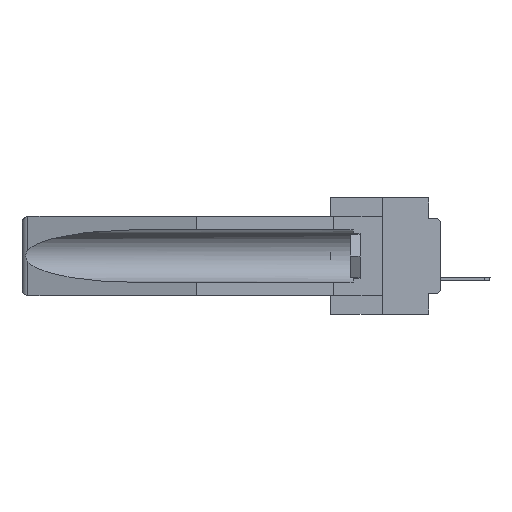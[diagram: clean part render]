
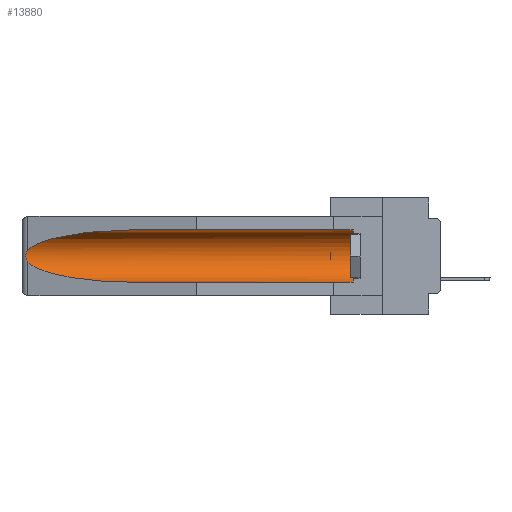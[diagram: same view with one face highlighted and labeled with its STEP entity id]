
A CAD part, left-side view. The second image highlights one B-rep face of the part: STEP entity #13880.
In plain terms, the highlighted cylindrical face has radius 2.857 mm (diameter 5.715 mm), a partial arc.
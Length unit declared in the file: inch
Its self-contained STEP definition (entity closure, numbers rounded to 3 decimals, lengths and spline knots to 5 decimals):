
#2899 = CARTESIAN_POINT ( 'NONE',  ( 0.26654, 1.53092, -0.15636 ) ) ;
#3730 = ORIENTED_EDGE ( 'NONE', *, *, #39658, .T. ) ;
#3812 = CARTESIAN_POINT ( 'NONE',  ( 0.155, -0.30754, -0.284 ) ) ;
#4003 = CARTESIAN_POINT ( 'NONE',  ( 0.155, 0.126, -0.1715 ) ) ;
#5681 = ORIENTED_EDGE ( 'NONE', *, *, #24620, .T. ) ;
#5721 = CARTESIAN_POINT ( 'NONE',  ( 0.2673, 1.53269, -0.17917 ) ) ;
#6647 = VERTEX_POINT ( 'NONE', #15003 ) ;
#6692 = FACE_OUTER_BOUND ( 'NONE', #24345, .T. ) ;
#7071 = VERTEX_POINT ( 'NONE', #22682 ) ;
#7233 = DIRECTION ( 'NONE',  ( 0., 0., 1. ) ) ;
#7911 = VECTOR ( 'NONE', #9457, 39.37008 ) ;
#8857 = VERTEX_POINT ( 'NONE', #20600 ) ;
#9457 = DIRECTION ( 'NONE',  ( 0., 1., 0. ) ) ;
#9599 =( BOUNDED_CURVE ( )  B_SPLINE_CURVE ( 3, ( #34732, #25431, #34131, #37180 ),
 .UNSPECIFIED., .F., .T. ) 
 B_SPLINE_CURVE_WITH_KNOTS ( ( 4, 4 ),
 ( 4.71239, 6.08839 ),
 .UNSPECIFIED. ) 
 CURVE ( )  GEOMETRIC_REPRESENTATION_ITEM ( )  RATIONAL_B_SPLINE_CURVE ( ( 1., 0.848, 0.848, 1. ) ) 
 REPRESENTATION_ITEM ( '' )  );
#9711 = EDGE_CURVE ( 'NONE', #28031, #6647, #16634, .T. ) ;
#10058 = DIRECTION ( 'NONE',  ( 0., -1., 0. ) ) ;
#12958 = VERTEX_POINT ( 'NONE', #27577 ) ;
#13326 = DIRECTION ( 'NONE',  ( 0., 1., 0. ) ) ;
#13880 = ADVANCED_FACE ( 'NONE', ( #6692 ), #16547, .F. ) ;
#14579 = CARTESIAN_POINT ( 'NONE',  ( 0.26597, 1.5296, -0.19026 ) ) ;
#14958 = VERTEX_POINT ( 'NONE', #20837 ) ;
#14965 = CARTESIAN_POINT ( 'NONE',  ( 0.26537, 1.52718, -0.14972 ) ) ;
#15003 = CARTESIAN_POINT ( 'NONE',  ( 0.26537, 1.52718, -0.19328 ) ) ;
#16547 = CYLINDRICAL_SURFACE ( 'NONE', #31322, 0.1125 ) ;
#16634 = B_SPLINE_CURVE_WITH_KNOTS ( 'NONE', 3,
 ( #14965, #39653, #2899, #27715, #36206, #24475, #5721, #18210, #14579, #30339 ),
 .UNSPECIFIED., .F., .F.,
 ( 4, 2, 2, 2, 4 ),
 ( 0., 0.00029, 0.00058, 0.00087, 0.00117 ),
 .UNSPECIFIED. ) ;
#16769 = CARTESIAN_POINT ( 'NONE',  ( 0.25451, 1.48313, -0.24835 ) ) ;
#17550 = CARTESIAN_POINT ( 'NONE',  ( 0.155, 1.07973, -0.284 ) ) ;
#18210 = CARTESIAN_POINT ( 'NONE',  ( 0.26655, 1.53094, -0.18657 ) ) ;
#19014 = AXIS2_PLACEMENT_3D ( 'NONE', #4003, #10058, #7233 ) ;
#19797 = DIRECTION ( 'NONE',  ( 0., 0., 1. ) ) ;
#19819 = EDGE_CURVE ( 'NONE', #6647, #12958, #28936, .T. ) ;
#20600 = CARTESIAN_POINT ( 'NONE',  ( 0.155, 0.126, -0.059 ) ) ;
#20837 = CARTESIAN_POINT ( 'NONE',  ( 0.155, 0.126, -0.284 ) ) ;
#21267 = ORIENTED_EDGE ( 'NONE', *, *, #19819, .T. ) ;
#21851 = ORIENTED_EDGE ( 'NONE', *, *, #25089, .F. ) ;
#22682 = CARTESIAN_POINT ( 'NONE',  ( 0.155, 1.07973, -0.059 ) ) ;
#24345 = EDGE_LOOP ( 'NONE', ( #29338, #39216, #21267, #21851, #3730, #5681 ) ) ;
#24475 = CARTESIAN_POINT ( 'NONE',  ( 0.2675, 1.53308, -0.17534 ) ) ;
#24620 = EDGE_CURVE ( 'NONE', #8857, #7071, #30903, .T. ) ;
#24633 = EDGE_CURVE ( 'NONE', #7071, #28031, #9599, .T. ) ;
#25089 = EDGE_CURVE ( 'NONE', #14958, #12958, #31462, .T. ) ;
#25431 = CARTESIAN_POINT ( 'NONE',  ( 0.21114, 1.30732, -0.059 ) ) ;
#27180 = CARTESIAN_POINT ( 'NONE',  ( 0.26537, 1.52718, -0.14972 ) ) ;
#27577 = CARTESIAN_POINT ( 'NONE',  ( 0.155, 1.07973, -0.284 ) ) ;
#27715 = CARTESIAN_POINT ( 'NONE',  ( 0.2673, 1.5327, -0.16383 ) ) ;
#28031 = VERTEX_POINT ( 'NONE', #27180 ) ;
#28936 =( BOUNDED_CURVE ( )  B_SPLINE_CURVE ( 3, ( #35358, #16769, #35759, #17550 ),
 .UNSPECIFIED., .F., .T. ) 
 B_SPLINE_CURVE_WITH_KNOTS ( ( 4, 4 ),
 ( 0.1948, 1.5708 ),
 .UNSPECIFIED. ) 
 CURVE ( )  GEOMETRIC_REPRESENTATION_ITEM ( )  RATIONAL_B_SPLINE_CURVE ( ( 1., 0.848, 0.848, 1. ) ) 
 REPRESENTATION_ITEM ( '' )  );
#29338 = ORIENTED_EDGE ( 'NONE', *, *, #24633, .T. ) ;
#30339 = CARTESIAN_POINT ( 'NONE',  ( 0.26537, 1.52718, -0.19328 ) ) ;
#30903 = LINE ( 'NONE', #31701, #36847 ) ;
#31322 = AXIS2_PLACEMENT_3D ( 'NONE', #38177, #34933, #19797 ) ;
#31462 = LINE ( 'NONE', #3812, #7911 ) ;
#31701 = CARTESIAN_POINT ( 'NONE',  ( 0.155, -0.30754, -0.059 ) ) ;
#34131 = CARTESIAN_POINT ( 'NONE',  ( 0.25451, 1.48313, -0.09465 ) ) ;
#34732 = CARTESIAN_POINT ( 'NONE',  ( 0.155, 1.07973, -0.059 ) ) ;
#34933 = DIRECTION ( 'NONE',  ( 0., 1., 0. ) ) ;
#35358 = CARTESIAN_POINT ( 'NONE',  ( 0.26537, 1.52718, -0.19328 ) ) ;
#35759 = CARTESIAN_POINT ( 'NONE',  ( 0.21114, 1.30732, -0.284 ) ) ;
#36206 = CARTESIAN_POINT ( 'NONE',  ( 0.2675, 1.53308, -0.16763 ) ) ;
#36416 = CIRCLE ( 'NONE', #19014, 0.1125 ) ;
#36847 = VECTOR ( 'NONE', #13326, 39.37008 ) ;
#37180 = CARTESIAN_POINT ( 'NONE',  ( 0.26537, 1.52718, -0.14972 ) ) ;
#38177 = CARTESIAN_POINT ( 'NONE',  ( 0.155, -0.30754, -0.1715 ) ) ;
#39216 = ORIENTED_EDGE ( 'NONE', *, *, #9711, .T. ) ;
#39653 = CARTESIAN_POINT ( 'NONE',  ( 0.26597, 1.52961, -0.15275 ) ) ;
#39658 = EDGE_CURVE ( 'NONE', #14958, #8857, #36416, .T. ) ;
